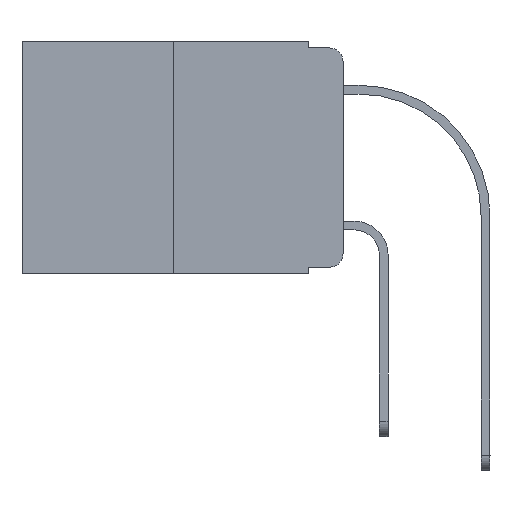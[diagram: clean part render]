
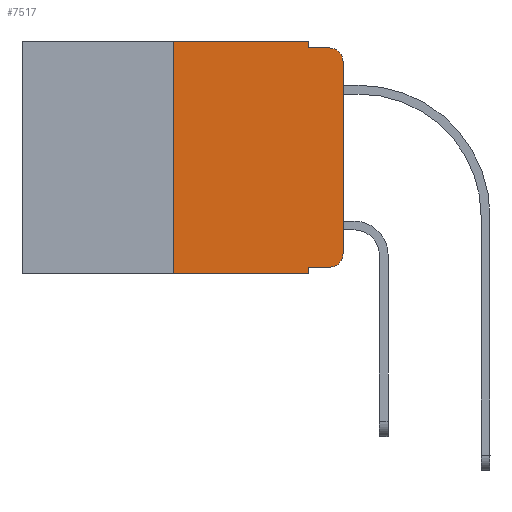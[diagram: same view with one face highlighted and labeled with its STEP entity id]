
A CAD part, left-side view. The second image highlights one B-rep face of the part: STEP entity #7517.
In plain terms, the highlighted planar face has unit normal (-1, 0, 0).
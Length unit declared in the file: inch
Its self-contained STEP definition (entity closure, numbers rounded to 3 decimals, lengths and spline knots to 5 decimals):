
#426 = DIRECTION ( 'NONE',  ( 0., 0., -1. ) ) ;
#542 = VERTEX_POINT ( 'NONE', #2042 ) ;
#567 = ORIENTED_EDGE ( 'NONE', *, *, #13498, .F. ) ;
#683 = DIRECTION ( 'NONE',  ( 1., 0., 0. ) ) ;
#834 = CARTESIAN_POINT ( 'NONE',  ( 0., 0.473, -0.343 ) ) ;
#1060 = LINE ( 'NONE', #18322, #1852 ) ;
#1540 = LINE ( 'NONE', #6206, #7159 ) ;
#1656 = EDGE_CURVE ( 'NONE', #10585, #7355, #1540, .T. ) ;
#1730 = VERTEX_POINT ( 'NONE', #15557 ) ;
#1852 = VECTOR ( 'NONE', #4209, 39.37008 ) ;
#2002 = PLANE ( 'NONE',  #11928 ) ;
#2042 = CARTESIAN_POINT ( 'NONE',  ( 0., 0.051, 0. ) ) ;
#2174 = VERTEX_POINT ( 'NONE', #3302 ) ;
#2676 = ORIENTED_EDGE ( 'NONE', *, *, #17728, .T. ) ;
#2984 = VERTEX_POINT ( 'NONE', #10177 ) ;
#3302 = CARTESIAN_POINT ( 'NONE',  ( 0., 0., -0.03 ) ) ;
#3535 = VECTOR ( 'NONE', #3893, 39.37008 ) ;
#3693 = CARTESIAN_POINT ( 'NONE',  ( 0., 0.02, -0.03 ) ) ;
#3718 = CARTESIAN_POINT ( 'NONE',  ( 0., 0.473, 0. ) ) ;
#3893 = DIRECTION ( 'NONE',  ( 0., -1., 0. ) ) ;
#3984 = EDGE_CURVE ( 'NONE', #2984, #2174, #4527, .T. ) ;
#3988 = LINE ( 'NONE', #834, #11760 ) ;
#4191 = LINE ( 'NONE', #5401, #3535 ) ;
#4205 = ORIENTED_EDGE ( 'NONE', *, *, #3984, .T. ) ;
#4209 = DIRECTION ( 'NONE',  ( 0., 0., -1. ) ) ;
#4527 = LINE ( 'NONE', #12242, #16509 ) ;
#5398 = VECTOR ( 'NONE', #14802, 39.37008 ) ;
#5401 = CARTESIAN_POINT ( 'NONE',  ( 0., 0.051, -0.01 ) ) ;
#5520 = DIRECTION ( 'NONE',  ( 0., -1., 0. ) ) ;
#5761 = ORIENTED_EDGE ( 'NONE', *, *, #15068, .T. ) ;
#5773 = EDGE_LOOP ( 'NONE', ( #4205, #2676, #6758, #9423, #567, #12100, #5761, #18543, #15822, #6245 ) ) ;
#6206 = CARTESIAN_POINT ( 'NONE',  ( 0., 0.25, 0. ) ) ;
#6245 = ORIENTED_EDGE ( 'NONE', *, *, #8002, .T. ) ;
#6758 = ORIENTED_EDGE ( 'NONE', *, *, #11393, .F. ) ;
#7159 = VECTOR ( 'NONE', #9167, 39.37008 ) ;
#7355 = VERTEX_POINT ( 'NONE', #9514 ) ;
#7517 = ADVANCED_FACE ( 'NONE', ( #11441 ), #2002, .F. ) ;
#7645 = AXIS2_PLACEMENT_3D ( 'NONE', #3693, #18316, #12019 ) ;
#8002 = EDGE_CURVE ( 'NONE', #1730, #2984, #15509, .T. ) ;
#8046 = AXIS2_PLACEMENT_3D ( 'NONE', #12726, #9692, #426 ) ;
#8564 = VERTEX_POINT ( 'NONE', #9207 ) ;
#8719 = LINE ( 'NONE', #14917, #5398 ) ;
#8932 = CARTESIAN_POINT ( 'NONE',  ( 0., 0.051, -0.01 ) ) ;
#9151 = CARTESIAN_POINT ( 'NONE',  ( 0., 0.051, -0.343 ) ) ;
#9167 = DIRECTION ( 'NONE',  ( 0., 0., 1. ) ) ;
#9207 = CARTESIAN_POINT ( 'NONE',  ( 0., 0.02, -0.01 ) ) ;
#9423 = ORIENTED_EDGE ( 'NONE', *, *, #9507, .F. ) ;
#9507 = EDGE_CURVE ( 'NONE', #542, #18251, #1060, .T. ) ;
#9514 = CARTESIAN_POINT ( 'NONE',  ( 0., 0.25, 0. ) ) ;
#9692 = DIRECTION ( 'NONE',  ( -1., 0., 0. ) ) ;
#10000 = CARTESIAN_POINT ( 'NONE',  ( 0., 0.051, -0.333 ) ) ;
#10177 = CARTESIAN_POINT ( 'NONE',  ( 0., 0., -0.313 ) ) ;
#10559 = CARTESIAN_POINT ( 'NONE',  ( 0., 0.25, -0.343 ) ) ;
#10585 = VERTEX_POINT ( 'NONE', #10559 ) ;
#11160 = VECTOR ( 'NONE', #19459, 39.37008 ) ;
#11346 = CARTESIAN_POINT ( 'NONE',  ( 0., 0.051, -0.333 ) ) ;
#11393 = EDGE_CURVE ( 'NONE', #18251, #8564, #4191, .T. ) ;
#11441 = FACE_OUTER_BOUND ( 'NONE', #5773, .T. ) ;
#11503 = EDGE_CURVE ( 'NONE', #13753, #15285, #13638, .T. ) ;
#11760 = VECTOR ( 'NONE', #5520, 39.37008 ) ;
#11928 = AXIS2_PLACEMENT_3D ( 'NONE', #3718, #683, #19487 ) ;
#12019 = DIRECTION ( 'NONE',  ( 0., 0., -1. ) ) ;
#12100 = ORIENTED_EDGE ( 'NONE', *, *, #1656, .F. ) ;
#12242 = CARTESIAN_POINT ( 'NONE',  ( 0., 0., 0. ) ) ;
#12726 = CARTESIAN_POINT ( 'NONE',  ( 0., 0.02, -0.313 ) ) ;
#13248 = LINE ( 'NONE', #10000, #11160 ) ;
#13498 = EDGE_CURVE ( 'NONE', #7355, #542, #8719, .T. ) ;
#13638 = LINE ( 'NONE', #19835, #14245 ) ;
#13753 = VERTEX_POINT ( 'NONE', #11346 ) ;
#14245 = VECTOR ( 'NONE', #19926, 39.37008 ) ;
#14297 = EDGE_CURVE ( 'NONE', #13753, #1730, #13248, .T. ) ;
#14802 = DIRECTION ( 'NONE',  ( 0., -1., 0. ) ) ;
#14917 = CARTESIAN_POINT ( 'NONE',  ( 0., 0.473, 0. ) ) ;
#15068 = EDGE_CURVE ( 'NONE', #10585, #15285, #3988, .T. ) ;
#15285 = VERTEX_POINT ( 'NONE', #9151 ) ;
#15293 = DIRECTION ( 'NONE',  ( 0., 0., 1. ) ) ;
#15509 = CIRCLE ( 'NONE', #8046, 0.02 ) ;
#15557 = CARTESIAN_POINT ( 'NONE',  ( 0., 0.02, -0.333 ) ) ;
#15822 = ORIENTED_EDGE ( 'NONE', *, *, #14297, .T. ) ;
#16423 = CIRCLE ( 'NONE', #7645, 0.02 ) ;
#16509 = VECTOR ( 'NONE', #15293, 39.37008 ) ;
#17728 = EDGE_CURVE ( 'NONE', #2174, #8564, #16423, .T. ) ;
#18251 = VERTEX_POINT ( 'NONE', #8932 ) ;
#18316 = DIRECTION ( 'NONE',  ( -1., 0., 0. ) ) ;
#18322 = CARTESIAN_POINT ( 'NONE',  ( 0., 0.051, 0. ) ) ;
#18543 = ORIENTED_EDGE ( 'NONE', *, *, #11503, .F. ) ;
#19459 = DIRECTION ( 'NONE',  ( 0., -1., 0. ) ) ;
#19487 = DIRECTION ( 'NONE',  ( 0., 0., -1. ) ) ;
#19835 = CARTESIAN_POINT ( 'NONE',  ( 0., 0.051, 0. ) ) ;
#19926 = DIRECTION ( 'NONE',  ( 0., 0., -1. ) ) ;
